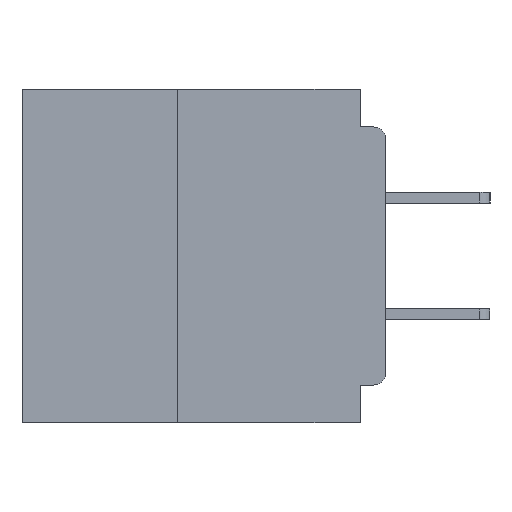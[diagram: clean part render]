
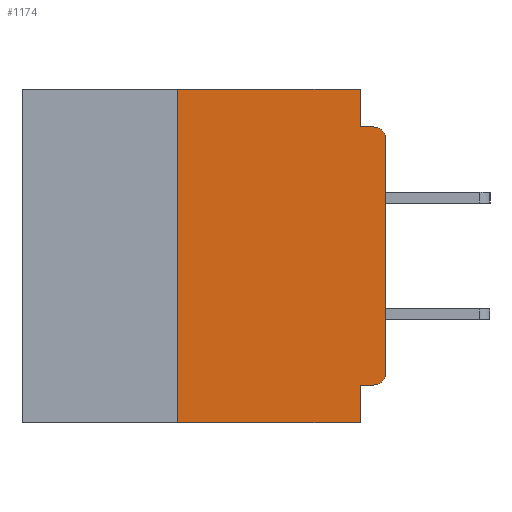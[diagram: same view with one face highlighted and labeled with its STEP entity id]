
A CAD part, left-side view. The second image highlights one B-rep face of the part: STEP entity #1174.
In plain terms, the highlighted planar face has unit normal (-1, 0, 0).
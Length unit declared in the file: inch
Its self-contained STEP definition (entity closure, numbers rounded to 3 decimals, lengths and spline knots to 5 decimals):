
#597 = VECTOR ( 'NONE', #2264, 39.37008 ) ;
#758 = VERTEX_POINT ( 'NONE', #2199 ) ;
#837 = ORIENTED_EDGE ( 'NONE', *, *, #16098, .F. ) ;
#975 = ORIENTED_EDGE ( 'NONE', *, *, #7134, .F. ) ;
#1174 = ADVANCED_FACE ( 'NONE', ( #12573 ), #36161, .F. ) ;
#1446 = ORIENTED_EDGE ( 'NONE', *, *, #21353, .T. ) ;
#1828 = CARTESIAN_POINT ( 'NONE',  ( 0., 0., -0.045 ) ) ;
#1997 = EDGE_CURVE ( 'NONE', #3275, #24726, #36706, .T. ) ;
#2199 = CARTESIAN_POINT ( 'NONE',  ( 0., 0.25, -0.4 ) ) ;
#2264 = DIRECTION ( 'NONE',  ( 0., -1., 0. ) ) ;
#2632 = ORIENTED_EDGE ( 'NONE', *, *, #25017, .T. ) ;
#3275 = VERTEX_POINT ( 'NONE', #8767 ) ;
#3326 = CARTESIAN_POINT ( 'NONE',  ( 0., 0.031, 0. ) ) ;
#4229 = CARTESIAN_POINT ( 'NONE',  ( 0., 0.015, -0.355 ) ) ;
#4782 = VERTEX_POINT ( 'NONE', #4229 ) ;
#5332 = ORIENTED_EDGE ( 'NONE', *, *, #5988, .F. ) ;
#5988 = EDGE_CURVE ( 'NONE', #31630, #22682, #27884, .T. ) ;
#6476 = CIRCLE ( 'NONE', #27462, 0.015 ) ;
#7073 = ORIENTED_EDGE ( 'NONE', *, *, #9672, .T. ) ;
#7134 = EDGE_CURVE ( 'NONE', #4782, #25765, #13041, .T. ) ;
#7756 = DIRECTION ( 'NONE',  ( -1., 0., 0. ) ) ;
#8767 = CARTESIAN_POINT ( 'NONE',  ( 0., 0.031, -0.045 ) ) ;
#9013 = AXIS2_PLACEMENT_3D ( 'NONE', #27539, #10353, #30385 ) ;
#9025 = DIRECTION ( 'NONE',  ( 0., 0., 1. ) ) ;
#9371 = CARTESIAN_POINT ( 'NONE',  ( 0., 0.25, -0.4 ) ) ;
#9672 = EDGE_CURVE ( 'NONE', #29584, #24726, #6476, .T. ) ;
#9797 = CARTESIAN_POINT ( 'NONE',  ( 0., 0., -0.06 ) ) ;
#10353 = DIRECTION ( 'NONE',  ( -1., 0., 0. ) ) ;
#10930 = CARTESIAN_POINT ( 'NONE',  ( 0., 0.031, -0.4 ) ) ;
#11219 = ORIENTED_EDGE ( 'NONE', *, *, #25648, .F. ) ;
#11790 = CARTESIAN_POINT ( 'NONE',  ( 0., 0., 0. ) ) ;
#11881 = VERTEX_POINT ( 'NONE', #20251 ) ;
#12042 = CARTESIAN_POINT ( 'NONE',  ( 0., 0.25, 0. ) ) ;
#12146 = LINE ( 'NONE', #24077, #26488 ) ;
#12476 = ORIENTED_EDGE ( 'NONE', *, *, #1997, .F. ) ;
#12573 = FACE_OUTER_BOUND ( 'NONE', #26747, .T. ) ;
#13041 = LINE ( 'NONE', #29658, #27337 ) ;
#13051 = ORIENTED_EDGE ( 'NONE', *, *, #36785, .T. ) ;
#13149 = AXIS2_PLACEMENT_3D ( 'NONE', #36168, #36094, #36056 ) ;
#13989 = DIRECTION ( 'NONE',  ( 0., 0., -1. ) ) ;
#14664 = VECTOR ( 'NONE', #13989, 39.37008 ) ;
#15442 = VECTOR ( 'NONE', #16332, 39.37008 ) ;
#16098 = EDGE_CURVE ( 'NONE', #22682, #3275, #30562, .T. ) ;
#16332 = DIRECTION ( 'NONE',  ( 0., 0., -1. ) ) ;
#18517 = DIRECTION ( 'NONE',  ( 0., -1., 0. ) ) ;
#19934 = LINE ( 'NONE', #9371, #34828 ) ;
#20251 = CARTESIAN_POINT ( 'NONE',  ( 0., 0.031, -0.4 ) ) ;
#20321 = VECTOR ( 'NONE', #33292, 39.37008 ) ;
#20531 = ORIENTED_EDGE ( 'NONE', *, *, #33171, .F. ) ;
#21353 = EDGE_CURVE ( 'NONE', #4782, #30852, #26856, .T. ) ;
#22238 = LINE ( 'NONE', #10930, #14664 ) ;
#22682 = VERTEX_POINT ( 'NONE', #3326 ) ;
#23889 = DIRECTION ( 'NONE',  ( 0., 1., 0. ) ) ;
#24077 = CARTESIAN_POINT ( 'NONE',  ( 0., 0.437, -0.4 ) ) ;
#24726 = VERTEX_POINT ( 'NONE', #30330 ) ;
#24802 = VECTOR ( 'NONE', #9025, 39.37008 ) ;
#24847 = CARTESIAN_POINT ( 'NONE',  ( 0., 0.437, 0. ) ) ;
#24931 = CARTESIAN_POINT ( 'NONE',  ( 0., 0.015, -0.06 ) ) ;
#25017 = EDGE_CURVE ( 'NONE', #30852, #29584, #32304, .T. ) ;
#25648 = EDGE_CURVE ( 'NONE', #758, #31630, #19934, .T. ) ;
#25765 = VERTEX_POINT ( 'NONE', #27042 ) ;
#26488 = VECTOR ( 'NONE', #18517, 39.37008 ) ;
#26747 = EDGE_LOOP ( 'NONE', ( #2632, #7073, #12476, #837, #5332, #11219, #13051, #20531, #975, #1446 ) ) ;
#26856 = CIRCLE ( 'NONE', #9013, 0.015 ) ;
#27042 = CARTESIAN_POINT ( 'NONE',  ( 0., 0.031, -0.355 ) ) ;
#27274 = CARTESIAN_POINT ( 'NONE',  ( 0., 0., -0.34 ) ) ;
#27337 = VECTOR ( 'NONE', #23889, 39.37008 ) ;
#27462 = AXIS2_PLACEMENT_3D ( 'NONE', #24931, #7756, #27810 ) ;
#27539 = CARTESIAN_POINT ( 'NONE',  ( 0., 0.015, -0.34 ) ) ;
#27644 = CARTESIAN_POINT ( 'NONE',  ( 0., 0.031, 0. ) ) ;
#27810 = DIRECTION ( 'NONE',  ( 0., 0., -1. ) ) ;
#27884 = LINE ( 'NONE', #24847, #20321 ) ;
#29443 = DIRECTION ( 'NONE',  ( 0., 0., 1. ) ) ;
#29584 = VERTEX_POINT ( 'NONE', #9797 ) ;
#29658 = CARTESIAN_POINT ( 'NONE',  ( 0., 0., -0.355 ) ) ;
#30330 = CARTESIAN_POINT ( 'NONE',  ( 0., 0.015, -0.045 ) ) ;
#30385 = DIRECTION ( 'NONE',  ( 0., 0., -1. ) ) ;
#30562 = LINE ( 'NONE', #27644, #15442 ) ;
#30852 = VERTEX_POINT ( 'NONE', #27274 ) ;
#31630 = VERTEX_POINT ( 'NONE', #12042 ) ;
#32304 = LINE ( 'NONE', #11790, #24802 ) ;
#33171 = EDGE_CURVE ( 'NONE', #25765, #11881, #22238, .T. ) ;
#33292 = DIRECTION ( 'NONE',  ( 0., -1., 0. ) ) ;
#34828 = VECTOR ( 'NONE', #29443, 39.37008 ) ;
#36056 = DIRECTION ( 'NONE',  ( 0., 0., -1. ) ) ;
#36094 = DIRECTION ( 'NONE',  ( 1., 0., 0. ) ) ;
#36161 = PLANE ( 'NONE',  #13149 ) ;
#36168 = CARTESIAN_POINT ( 'NONE',  ( 0., 0.437, 0. ) ) ;
#36706 = LINE ( 'NONE', #1828, #597 ) ;
#36785 = EDGE_CURVE ( 'NONE', #758, #11881, #12146, .T. ) ;
